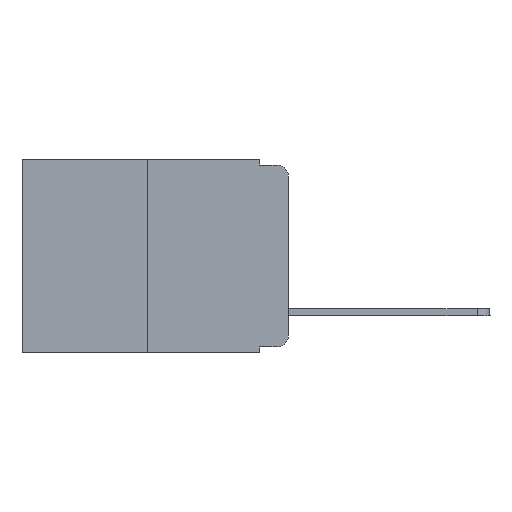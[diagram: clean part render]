
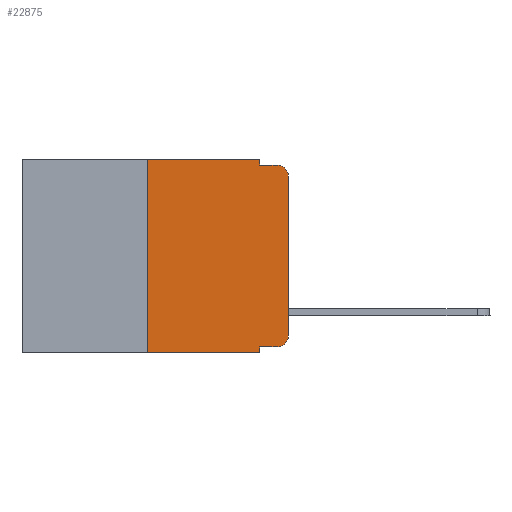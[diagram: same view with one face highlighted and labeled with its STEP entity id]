
A CAD part, left-side view. The second image highlights one B-rep face of the part: STEP entity #22875.
In plain terms, the highlighted planar face has unit normal (-1, 0, 0).
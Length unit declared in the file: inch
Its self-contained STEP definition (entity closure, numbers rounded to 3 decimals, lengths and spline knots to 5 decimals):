
#97 = AXIS2_PLACEMENT_3D ( 'NONE', #1835, #5866, #9707 ) ;
#250 = EDGE_CURVE ( 'NONE', #25425, #24374, #25535, .T. ) ;
#264 = VERTEX_POINT ( 'NONE', #4034 ) ;
#304 = CARTESIAN_POINT ( 'NONE',  ( 0., 0.473, 0. ) ) ;
#1835 = CARTESIAN_POINT ( 'NONE',  ( 0., 0.02, -0.03 ) ) ;
#1925 = DIRECTION ( 'NONE',  ( 0., 0., -1. ) ) ;
#2345 = CARTESIAN_POINT ( 'NONE',  ( 0., 0.051, -0.333 ) ) ;
#2405 = LINE ( 'NONE', #11890, #6149 ) ;
#2590 = CARTESIAN_POINT ( 'NONE',  ( 0., 0.25, 0. ) ) ;
#2733 = EDGE_CURVE ( 'NONE', #8285, #4074, #15890, .T. ) ;
#3019 = CARTESIAN_POINT ( 'NONE',  ( 0., 0.02, -0.01 ) ) ;
#3339 = EDGE_CURVE ( 'NONE', #16159, #16043, #4206, .T. ) ;
#3416 = ORIENTED_EDGE ( 'NONE', *, *, #9616, .F. ) ;
#3695 = CARTESIAN_POINT ( 'NONE',  ( 0., 0.051, 0. ) ) ;
#3803 = CARTESIAN_POINT ( 'NONE',  ( 0., 0.02, -0.333 ) ) ;
#4034 = CARTESIAN_POINT ( 'NONE',  ( 0., 0.25, -0.343 ) ) ;
#4074 = VERTEX_POINT ( 'NONE', #3019 ) ;
#4206 = LINE ( 'NONE', #304, #14312 ) ;
#4336 = CARTESIAN_POINT ( 'NONE',  ( 0., 0.473, -0.343 ) ) ;
#4448 = ORIENTED_EDGE ( 'NONE', *, *, #2733, .F. ) ;
#4895 = VECTOR ( 'NONE', #1925, 39.37008 ) ;
#4975 = EDGE_LOOP ( 'NONE', ( #9635, #16322, #4448, #3416, #21940, #9142, #25020, #16869, #5312, #17382 ) ) ;
#5312 = ORIENTED_EDGE ( 'NONE', *, *, #15977, .T. ) ;
#5693 = DIRECTION ( 'NONE',  ( 0., 0., 1. ) ) ;
#5849 = CARTESIAN_POINT ( 'NONE',  ( 0., 0.051, -0.333 ) ) ;
#5866 = DIRECTION ( 'NONE',  ( -1., 0., 0. ) ) ;
#6149 = VECTOR ( 'NONE', #17707, 39.37008 ) ;
#6915 = CIRCLE ( 'NONE', #16047, 0.02 ) ;
#7628 = VECTOR ( 'NONE', #16512, 39.37008 ) ;
#7662 = CARTESIAN_POINT ( 'NONE',  ( 0., 0.051, 0. ) ) ;
#8285 = VERTEX_POINT ( 'NONE', #25696 ) ;
#8352 = VECTOR ( 'NONE', #13345, 39.37008 ) ;
#8437 = CARTESIAN_POINT ( 'NONE',  ( 0., 0.051, -0.343 ) ) ;
#8606 = PLANE ( 'NONE',  #12676 ) ;
#8898 = VERTEX_POINT ( 'NONE', #5849 ) ;
#8979 = EDGE_CURVE ( 'NONE', #264, #16159, #2405, .T. ) ;
#9061 = CARTESIAN_POINT ( 'NONE',  ( 0., 0., -0.03 ) ) ;
#9142 = ORIENTED_EDGE ( 'NONE', *, *, #8979, .F. ) ;
#9405 = LINE ( 'NONE', #2345, #22008 ) ;
#9616 = EDGE_CURVE ( 'NONE', #16043, #8285, #19067, .T. ) ;
#9635 = ORIENTED_EDGE ( 'NONE', *, *, #250, .T. ) ;
#9707 = DIRECTION ( 'NONE',  ( 0., 0., -1. ) ) ;
#10457 = EDGE_CURVE ( 'NONE', #24374, #4074, #16823, .T. ) ;
#11410 = FACE_OUTER_BOUND ( 'NONE', #4975, .T. ) ;
#11890 = CARTESIAN_POINT ( 'NONE',  ( 0., 0.25, 0. ) ) ;
#12676 = AXIS2_PLACEMENT_3D ( 'NONE', #22700, #20406, #18463 ) ;
#13345 = DIRECTION ( 'NONE',  ( 0., 0., -1. ) ) ;
#13398 = EDGE_CURVE ( 'NONE', #264, #19283, #18983, .T. ) ;
#14312 = VECTOR ( 'NONE', #18394, 39.37008 ) ;
#14563 = EDGE_CURVE ( 'NONE', #23227, #25425, #6915, .T. ) ;
#15340 = CARTESIAN_POINT ( 'NONE',  ( 0., 0., -0.313 ) ) ;
#15890 = LINE ( 'NONE', #18857, #17486 ) ;
#15977 = EDGE_CURVE ( 'NONE', #8898, #23227, #9405, .T. ) ;
#16043 = VERTEX_POINT ( 'NONE', #20941 ) ;
#16047 = AXIS2_PLACEMENT_3D ( 'NONE', #25356, #17323, #19337 ) ;
#16159 = VERTEX_POINT ( 'NONE', #2590 ) ;
#16322 = ORIENTED_EDGE ( 'NONE', *, *, #10457, .T. ) ;
#16512 = DIRECTION ( 'NONE',  ( 0., -1., 0. ) ) ;
#16823 = CIRCLE ( 'NONE', #97, 0.02 ) ;
#16869 = ORIENTED_EDGE ( 'NONE', *, *, #17157, .F. ) ;
#17157 = EDGE_CURVE ( 'NONE', #8898, #19283, #19459, .T. ) ;
#17323 = DIRECTION ( 'NONE',  ( -1., 0., 0. ) ) ;
#17382 = ORIENTED_EDGE ( 'NONE', *, *, #14563, .T. ) ;
#17486 = VECTOR ( 'NONE', #24699, 39.37008 ) ;
#17707 = DIRECTION ( 'NONE',  ( 0., 0., 1. ) ) ;
#18299 = DIRECTION ( 'NONE',  ( 0., -1., 0. ) ) ;
#18394 = DIRECTION ( 'NONE',  ( 0., -1., 0. ) ) ;
#18463 = DIRECTION ( 'NONE',  ( 0., 0., -1. ) ) ;
#18857 = CARTESIAN_POINT ( 'NONE',  ( 0., 0.051, -0.01 ) ) ;
#18983 = LINE ( 'NONE', #4336, #7628 ) ;
#19067 = LINE ( 'NONE', #7662, #8352 ) ;
#19283 = VERTEX_POINT ( 'NONE', #8437 ) ;
#19337 = DIRECTION ( 'NONE',  ( 0., 0., -1. ) ) ;
#19459 = LINE ( 'NONE', #3695, #4895 ) ;
#19571 = CARTESIAN_POINT ( 'NONE',  ( 0., 0., 0. ) ) ;
#20406 = DIRECTION ( 'NONE',  ( 1., 0., 0. ) ) ;
#20470 = VECTOR ( 'NONE', #5693, 39.37008 ) ;
#20941 = CARTESIAN_POINT ( 'NONE',  ( 0., 0.051, 0. ) ) ;
#21940 = ORIENTED_EDGE ( 'NONE', *, *, #3339, .F. ) ;
#22008 = VECTOR ( 'NONE', #18299, 39.37008 ) ;
#22700 = CARTESIAN_POINT ( 'NONE',  ( 0., 0.473, 0. ) ) ;
#22875 = ADVANCED_FACE ( 'NONE', ( #11410 ), #8606, .F. ) ;
#23227 = VERTEX_POINT ( 'NONE', #3803 ) ;
#24374 = VERTEX_POINT ( 'NONE', #9061 ) ;
#24699 = DIRECTION ( 'NONE',  ( 0., -1., 0. ) ) ;
#25020 = ORIENTED_EDGE ( 'NONE', *, *, #13398, .T. ) ;
#25356 = CARTESIAN_POINT ( 'NONE',  ( 0., 0.02, -0.313 ) ) ;
#25425 = VERTEX_POINT ( 'NONE', #15340 ) ;
#25535 = LINE ( 'NONE', #19571, #20470 ) ;
#25696 = CARTESIAN_POINT ( 'NONE',  ( 0., 0.051, -0.01 ) ) ;
